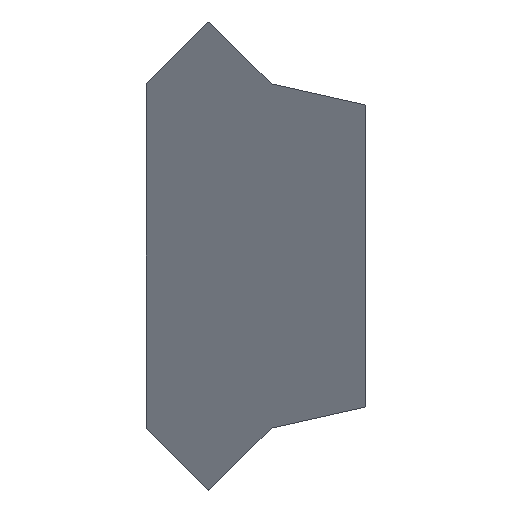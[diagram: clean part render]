
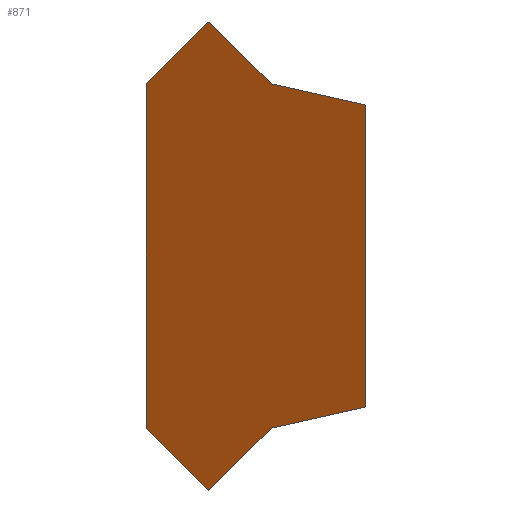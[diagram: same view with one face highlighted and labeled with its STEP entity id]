
A CAD part, front view. The second image highlights one B-rep face of the part: STEP entity #871.
In plain terms, the highlighted planar face has unit normal (-0.575, -0.818, 0).
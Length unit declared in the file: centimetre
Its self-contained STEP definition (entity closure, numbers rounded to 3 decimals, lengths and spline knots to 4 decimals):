
#99=FACE_OUTER_BOUND($,#161,.T.);
#161=EDGE_LOOP($,(#663,#664,#665,#666,#667,#668,#669,#670));
#192=LINE($,#1200,#276);
#216=LINE($,#1617,#300);
#217=LINE($,#1619,#301);
#218=LINE($,#1621,#302);
#219=LINE($,#1623,#303);
#220=LINE($,#1625,#304);
#221=LINE($,#1627,#305);
#222=LINE($,#1628,#306);
#276=VECTOR($,#977,1.4228);
#300=VECTOR($,#1077,0.5543);
#301=VECTOR($,#1078,0.5543);
#302=VECTOR($,#1079,0.4626);
#303=VECTOR($,#1080,0.4626);
#304=VECTOR($,#1081,1.6225);
#305=VECTOR($,#1082,0.4626);
#306=VECTOR($,#1083,0.4626);
#359=VERTEX_POINT($,#1196);
#361=VERTEX_POINT($,#1199);
#411=VERTEX_POINT($,#1616);
#412=VERTEX_POINT($,#1618);
#413=VERTEX_POINT($,#1620);
#414=VERTEX_POINT($,#1622);
#415=VERTEX_POINT($,#1624);
#416=VERTEX_POINT($,#1626);
#440=EDGE_CURVE($,#359,#361,#192,.T.);
#504=EDGE_CURVE($,#361,#411,#216,.T.);
#505=EDGE_CURVE($,#412,#359,#217,.T.);
#506=EDGE_CURVE($,#413,#412,#218,.T.);
#507=EDGE_CURVE($,#414,#413,#219,.T.);
#508=EDGE_CURVE($,#415,#414,#220,.T.);
#509=EDGE_CURVE($,#416,#415,#221,.T.);
#510=EDGE_CURVE($,#411,#416,#222,.T.);
#663=ORIENTED_EDGE($,*,*,#504,.F.);
#664=ORIENTED_EDGE($,*,*,#440,.F.);
#665=ORIENTED_EDGE($,*,*,#505,.F.);
#666=ORIENTED_EDGE($,*,*,#506,.F.);
#667=ORIENTED_EDGE($,*,*,#507,.F.);
#668=ORIENTED_EDGE($,*,*,#508,.F.);
#669=ORIENTED_EDGE($,*,*,#509,.F.);
#670=ORIENTED_EDGE($,*,*,#510,.F.);
#819=PLANE($,#942);
#871=ADVANCED_FACE($,(#99),#819,.F.);
#942=AXIS2_PLACEMENT_3D($,#1615,#1075,#1076);
#977=DIRECTION($,(0.,0.,-1.));
#1075=DIRECTION('center_axis',(0.575,0.818,0.));
#1076=DIRECTION('ref_axis',(-0.669,0.471,-0.575));
#1077=DIRECTION($,(-0.805,0.566,-0.18));
#1078=DIRECTION($,(0.805,-0.566,-0.18));
#1079=DIRECTION($,(0.636,-0.447,-0.63));
#1080=DIRECTION($,(0.636,-0.447,0.63));
#1081=DIRECTION($,(0.,0.,1.));
#1082=DIRECTION($,(-0.636,0.447,0.63));
#1083=DIRECTION($,(-0.636,0.447,-0.63));
#1196=CARTESIAN_POINT('',(-25.2982,1.373,0.8114));
#1199=CARTESIAN_POINT('',(-25.2982,1.373,-0.6114));
#1200=CARTESIAN_POINT($,(-25.2982,1.373,0.1047));
#1615=CARTESIAN_POINT('Origin',(-24.5968,0.8798,0.1094));
#1616=CARTESIAN_POINT('',(-25.7442,1.6866,-0.7113));
#1617=CARTESIAN_POINT($,(-24.7705,1.002,-0.4933));
#1618=CARTESIAN_POINT('',(-25.7442,1.6866,0.9113));
#1619=CARTESIAN_POINT($,(-24.7719,1.0029,0.6936));
#1620=CARTESIAN_POINT('',(-26.0382,1.8933,1.2025));
#1621=CARTESIAN_POINT($,(-25.0852,1.2233,0.2585));
#1622=CARTESIAN_POINT('',(-26.3322,2.1,0.9113));
#1623=CARTESIAN_POINT($,(-28.3243,3.5007,-1.062));
#1624=CARTESIAN_POINT('',(-26.3322,2.1,-0.7113));
#1625=CARTESIAN_POINT($,(-26.3322,2.1,0.1047));
#1626=CARTESIAN_POINT('',(-26.0382,1.8933,-1.0025));
#1627=CARTESIAN_POINT($,(-28.328,3.5034,1.2657));
#1628=CARTESIAN_POINT($,(-25.0815,1.2206,-0.0548));
